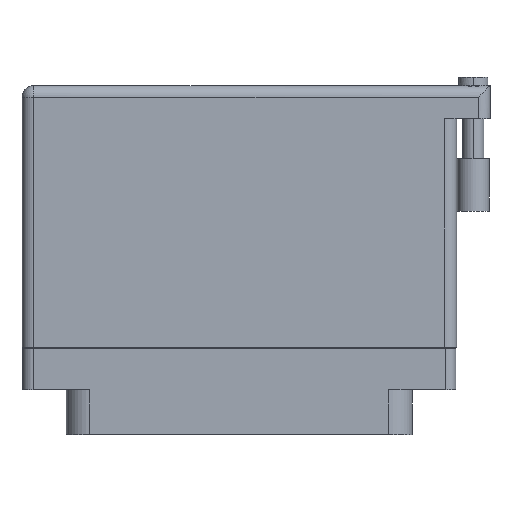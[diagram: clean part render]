
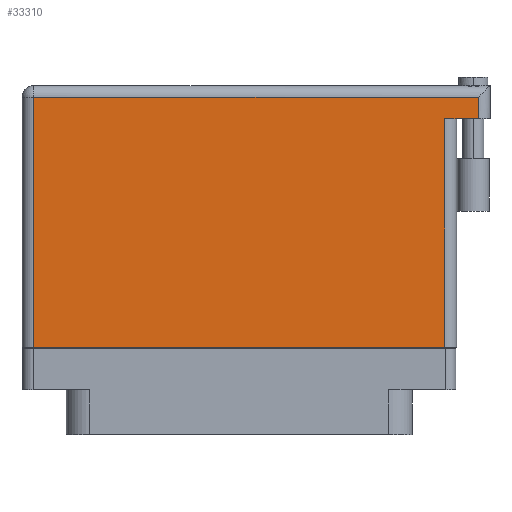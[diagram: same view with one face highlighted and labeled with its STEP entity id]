
A CAD part, front view. The second image highlights one B-rep face of the part: STEP entity #33310.
In plain terms, the highlighted face is planar.
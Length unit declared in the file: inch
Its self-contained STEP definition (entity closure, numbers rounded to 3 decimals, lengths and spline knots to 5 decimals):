
#391 = CARTESIAN_POINT ( 'NONE',  ( -1.3, -0.1, 0.4495 ) ) ;
#1339 = EDGE_CURVE ( 'NONE', #4579, #31062, #26769, .T. ) ;
#2794 = CARTESIAN_POINT ( 'NONE',  ( 1.5, 1.269, 0.4495 ) ) ;
#3074 = VECTOR ( 'NONE', #32325, 39.37008 ) ;
#3781 = EDGE_CURVE ( 'NONE', #50268, #27858, #11443, .T. ) ;
#4579 = VERTEX_POINT ( 'NONE', #15711 ) ;
#4744 = CARTESIAN_POINT ( 'NONE',  ( 1.43, 1.396, 0.4495 ) ) ;
#9012 = DIRECTION ( 'NONE',  ( 1., 0., 0. ) ) ;
#9303 = VECTOR ( 'NONE', #9012, 39.37008 ) ;
#10224 = ORIENTED_EDGE ( 'NONE', *, *, #3781, .T. ) ;
#10598 = EDGE_LOOP ( 'NONE', ( #39749, #10224, #15853, #34597, #10984, #13590 ) ) ;
#10984 = ORIENTED_EDGE ( 'NONE', *, *, #27842, .T. ) ;
#11443 = LINE ( 'NONE', #51566, #46890 ) ;
#11585 = LINE ( 'NONE', #2794, #38960 ) ;
#13590 = ORIENTED_EDGE ( 'NONE', *, *, #1339, .T. ) ;
#14006 = LINE ( 'NONE', #25823, #14659 ) ;
#14150 = DIRECTION ( 'NONE',  ( -1., 0., 0. ) ) ;
#14659 = VECTOR ( 'NONE', #14150, 39.37008 ) ;
#14972 = VECTOR ( 'NONE', #48610, 39.37008 ) ;
#15514 = PLANE ( 'NONE',  #42266 ) ;
#15711 = CARTESIAN_POINT ( 'NONE',  ( -1.23, 1.396, 0.4495 ) ) ;
#15853 = ORIENTED_EDGE ( 'NONE', *, *, #44621, .F. ) ;
#16025 = DIRECTION ( 'NONE',  ( 0., 0., -1. ) ) ;
#16270 = FACE_OUTER_BOUND ( 'NONE', #10598, .T. ) ;
#20642 = CARTESIAN_POINT ( 'NONE',  ( -1.23, -0.1, 0.4495 ) ) ;
#20663 = CARTESIAN_POINT ( 'NONE',  ( 1.23, -0.1, 0.4495 ) ) ;
#22505 = DIRECTION ( 'NONE',  ( -1., 0., 0. ) ) ;
#25274 = CARTESIAN_POINT ( 'NONE',  ( -1.23, -0.1, 0.4495 ) ) ;
#25823 = CARTESIAN_POINT ( 'NONE',  ( -1.3, 1.396, 0.4495 ) ) ;
#26162 = CARTESIAN_POINT ( 'NONE',  ( 1.23, 1.269, 0.4495 ) ) ;
#26769 = LINE ( 'NONE', #20642, #3074 ) ;
#27771 = DIRECTION ( 'NONE',  ( 0., 1., 0. ) ) ;
#27842 = EDGE_CURVE ( 'NONE', #33702, #4579, #14006, .T. ) ;
#27858 = VERTEX_POINT ( 'NONE', #26162 ) ;
#28041 = LINE ( 'NONE', #44674, #14972 ) ;
#31062 = VERTEX_POINT ( 'NONE', #25274 ) ;
#32325 = DIRECTION ( 'NONE',  ( 0., -1., 0. ) ) ;
#33265 = VERTEX_POINT ( 'NONE', #36233 ) ;
#33310 = ADVANCED_FACE ( 'NONE', ( #16270 ), #15514, .F. ) ;
#33702 = VERTEX_POINT ( 'NONE', #4744 ) ;
#34597 = ORIENTED_EDGE ( 'NONE', *, *, #46269, .T. ) ;
#35555 = CARTESIAN_POINT ( 'NONE',  ( -1.3, 1.466, 0.4495 ) ) ;
#36233 = CARTESIAN_POINT ( 'NONE',  ( 1.43, 1.269, 0.4495 ) ) ;
#36691 = LINE ( 'NONE', #391, #9303 ) ;
#38960 = VECTOR ( 'NONE', #22505, 39.37008 ) ;
#39749 = ORIENTED_EDGE ( 'NONE', *, *, #43069, .T. ) ;
#42266 = AXIS2_PLACEMENT_3D ( 'NONE', #35555, #16025, #51636 ) ;
#43069 = EDGE_CURVE ( 'NONE', #31062, #50268, #36691, .T. ) ;
#44621 = EDGE_CURVE ( 'NONE', #33265, #27858, #11585, .T. ) ;
#44674 = CARTESIAN_POINT ( 'NONE',  ( 1.43, 1.466, 0.4495 ) ) ;
#46269 = EDGE_CURVE ( 'NONE', #33265, #33702, #28041, .T. ) ;
#46890 = VECTOR ( 'NONE', #27771, 39.37008 ) ;
#48610 = DIRECTION ( 'NONE',  ( 0., 1., 0. ) ) ;
#50268 = VERTEX_POINT ( 'NONE', #20663 ) ;
#51566 = CARTESIAN_POINT ( 'NONE',  ( 1.23, 1.269, 0.4495 ) ) ;
#51636 = DIRECTION ( 'NONE',  ( -1., 0., 0. ) ) ;
